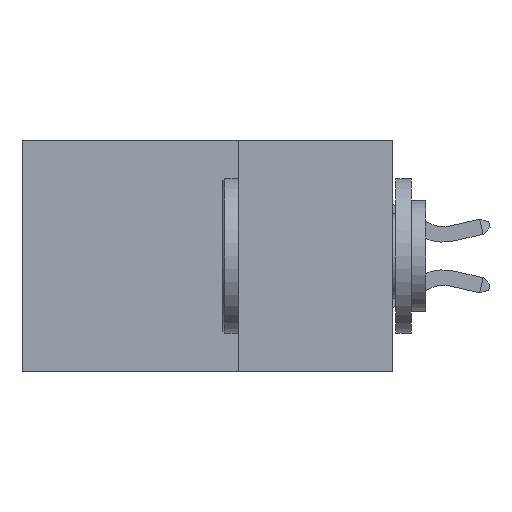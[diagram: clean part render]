
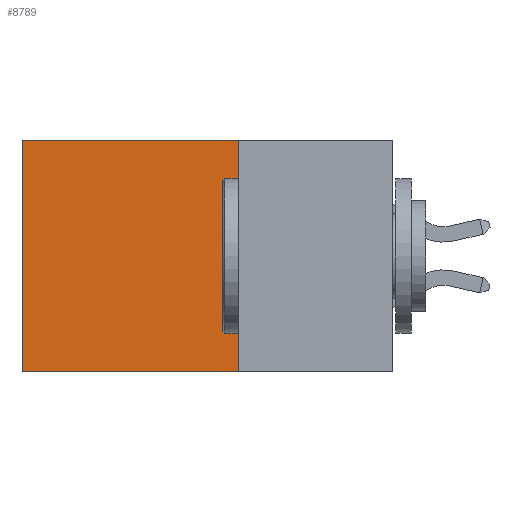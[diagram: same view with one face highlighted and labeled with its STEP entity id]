
A CAD part, left-side view. The second image highlights one B-rep face of the part: STEP entity #8789.
In plain terms, the highlighted planar face has unit normal (-1, 0, 0).
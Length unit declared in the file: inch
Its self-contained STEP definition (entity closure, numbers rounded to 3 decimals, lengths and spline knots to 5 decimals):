
#7 = DIRECTION ( 'NONE',  ( 0., 0., -1. ) ) ;
#44 = VERTEX_POINT ( 'NONE', #3064 ) ;
#94 = AXIS2_PLACEMENT_3D ( 'NONE', #4508, #8119, #7 ) ;
#320 = LINE ( 'NONE', #6745, #6577 ) ;
#531 = CARTESIAN_POINT ( 'NONE',  ( 0.2875, 0.25, -0.375 ) ) ;
#855 = VERTEX_POINT ( 'NONE', #7805 ) ;
#1424 = EDGE_LOOP ( 'NONE', ( #9031, #5289, #3932, #2974 ) ) ;
#1688 = VECTOR ( 'NONE', #3349, 39.37008 ) ;
#2038 = CARTESIAN_POINT ( 'NONE',  ( 0.2875, 0.25, -0.375 ) ) ;
#2232 = PLANE ( 'NONE',  #94 ) ;
#2396 = CARTESIAN_POINT ( 'NONE',  ( 0.2875, 0.25, 0. ) ) ;
#2719 = VECTOR ( 'NONE', #3531, 39.37008 ) ;
#2807 = EDGE_CURVE ( 'NONE', #4242, #4657, #8872, .T. ) ;
#2974 = ORIENTED_EDGE ( 'NONE', *, *, #5557, .T. ) ;
#3019 = EDGE_CURVE ( 'NONE', #4657, #44, #4924, .T. ) ;
#3064 = CARTESIAN_POINT ( 'NONE',  ( 0.2875, 0.6, -0.375 ) ) ;
#3349 = DIRECTION ( 'NONE',  ( 0., 1., 0. ) ) ;
#3531 = DIRECTION ( 'NONE',  ( 0., 1., 0. ) ) ;
#3932 = ORIENTED_EDGE ( 'NONE', *, *, #2807, .F. ) ;
#4242 = VERTEX_POINT ( 'NONE', #2396 ) ;
#4508 = CARTESIAN_POINT ( 'NONE',  ( 0.2875, 0.25, -0.375 ) ) ;
#4583 = VECTOR ( 'NONE', #5627, 39.37008 ) ;
#4591 = DIRECTION ( 'NONE',  ( 0., 0., -1. ) ) ;
#4657 = VERTEX_POINT ( 'NONE', #2038 ) ;
#4924 = LINE ( 'NONE', #7966, #2719 ) ;
#5056 = EDGE_CURVE ( 'NONE', #855, #44, #320, .T. ) ;
#5289 = ORIENTED_EDGE ( 'NONE', *, *, #3019, .F. ) ;
#5557 = EDGE_CURVE ( 'NONE', #4242, #855, #8290, .T. ) ;
#5627 = DIRECTION ( 'NONE',  ( 0., 0., -1. ) ) ;
#6266 = CARTESIAN_POINT ( 'NONE',  ( 0.2875, 0.25, 0. ) ) ;
#6577 = VECTOR ( 'NONE', #4591, 39.37008 ) ;
#6745 = CARTESIAN_POINT ( 'NONE',  ( 0.2875, 0.6, -0.375 ) ) ;
#7805 = CARTESIAN_POINT ( 'NONE',  ( 0.2875, 0.6, 0. ) ) ;
#7966 = CARTESIAN_POINT ( 'NONE',  ( 0.2875, 0.25, -0.375 ) ) ;
#8119 = DIRECTION ( 'NONE',  ( 1., 0., 0. ) ) ;
#8290 = LINE ( 'NONE', #6266, #1688 ) ;
#8789 = ADVANCED_FACE ( 'NONE', ( #9372 ), #2232, .F. ) ;
#8872 = LINE ( 'NONE', #531, #4583 ) ;
#9031 = ORIENTED_EDGE ( 'NONE', *, *, #5056, .T. ) ;
#9372 = FACE_OUTER_BOUND ( 'NONE', #1424, .T. ) ;
